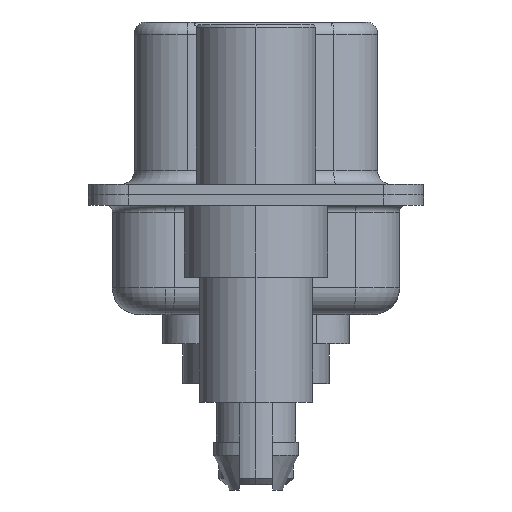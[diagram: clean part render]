
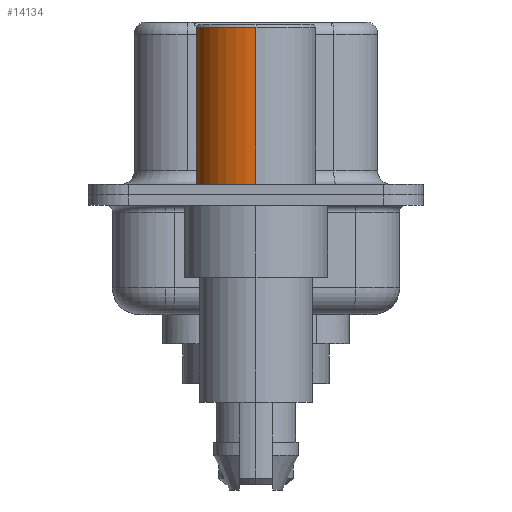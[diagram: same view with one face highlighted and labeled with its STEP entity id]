
A CAD part, left-side view. The second image highlights one B-rep face of the part: STEP entity #14134.
In plain terms, the highlighted cylindrical face has radius 2.25 mm (diameter 4.5 mm), a partial arc.
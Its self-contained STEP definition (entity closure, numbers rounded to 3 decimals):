
#40 = EDGE_CURVE ( 'NONE', #343, #8225, #12020, .T. ) ;
#336 = VECTOR ( 'NONE', #373, 1000. ) ;
#343 = VERTEX_POINT ( 'NONE', #1955 ) ;
#373 = DIRECTION ( 'NONE',  ( 0., 0., 1. ) ) ;
#637 = VECTOR ( 'NONE', #7717, 1000. ) ;
#1556 = CARTESIAN_POINT ( 'NONE',  ( -2.25, 0., 0.581 ) ) ;
#1747 = VERTEX_POINT ( 'NONE', #13338 ) ;
#1860 = DIRECTION ( 'NONE',  ( 0., 0., 1. ) ) ;
#1955 = CARTESIAN_POINT ( 'NONE',  ( -2.25, 0., 0.4 ) ) ;
#2094 = CARTESIAN_POINT ( 'NONE',  ( 0., 0., 0.581 ) ) ;
#2165 = CARTESIAN_POINT ( 'NONE',  ( 2.25, 0., 0.581 ) ) ;
#3143 = DIRECTION ( 'NONE',  ( 1., 0., 0. ) ) ;
#5152 = LINE ( 'NONE', #2165, #637 ) ;
#5263 = DIRECTION ( 'NONE',  ( 1., 0., 0. ) ) ;
#6017 = EDGE_CURVE ( 'NONE', #1747, #343, #15621, .T. ) ;
#6052 = ORIENTED_EDGE ( 'NONE', *, *, #40, .T. ) ;
#6084 = DIRECTION ( 'NONE',  ( 1., 0., 0. ) ) ;
#6363 = DIRECTION ( 'NONE',  ( 0., 0., 1. ) ) ;
#6432 = ORIENTED_EDGE ( 'NONE', *, *, #6017, .T. ) ;
#6823 = CARTESIAN_POINT ( 'NONE',  ( 0., 0., 6.3 ) ) ;
#7084 = AXIS2_PLACEMENT_3D ( 'NONE', #12878, #6363, #5263 ) ;
#7717 = DIRECTION ( 'NONE',  ( 0., 0., 1. ) ) ;
#8069 = EDGE_CURVE ( 'NONE', #12194, #8225, #9136, .T. ) ;
#8225 = VERTEX_POINT ( 'NONE', #15131 ) ;
#9041 = EDGE_CURVE ( 'NONE', #1747, #12194, #5152, .T. ) ;
#9136 = CIRCLE ( 'NONE', #14493, 2.25 ) ;
#9964 = CYLINDRICAL_SURFACE ( 'NONE', #13400, 2.25 ) ;
#11536 = ORIENTED_EDGE ( 'NONE', *, *, #8069, .F. ) ;
#12020 = LINE ( 'NONE', #1556, #336 ) ;
#12194 = VERTEX_POINT ( 'NONE', #12792 ) ;
#12294 = DIRECTION ( 'NONE',  ( 0., 0., 1. ) ) ;
#12792 = CARTESIAN_POINT ( 'NONE',  ( 2.25, 0., 6.3 ) ) ;
#12819 = ORIENTED_EDGE ( 'NONE', *, *, #9041, .F. ) ;
#12878 = CARTESIAN_POINT ( 'NONE',  ( 0., 0., 0.4 ) ) ;
#13338 = CARTESIAN_POINT ( 'NONE',  ( 2.25, 0., 0.4 ) ) ;
#13400 = AXIS2_PLACEMENT_3D ( 'NONE', #2094, #12294, #6084 ) ;
#14069 = EDGE_LOOP ( 'NONE', ( #6432, #6052, #11536, #12819 ) ) ;
#14134 = ADVANCED_FACE ( 'NONE', ( #14775 ), #9964, .T. ) ;
#14493 = AXIS2_PLACEMENT_3D ( 'NONE', #6823, #1860, #3143 ) ;
#14775 = FACE_OUTER_BOUND ( 'NONE', #14069, .T. ) ;
#15131 = CARTESIAN_POINT ( 'NONE',  ( -2.25, 0., 6.3 ) ) ;
#15621 = CIRCLE ( 'NONE', #7084, 2.25 ) ;
